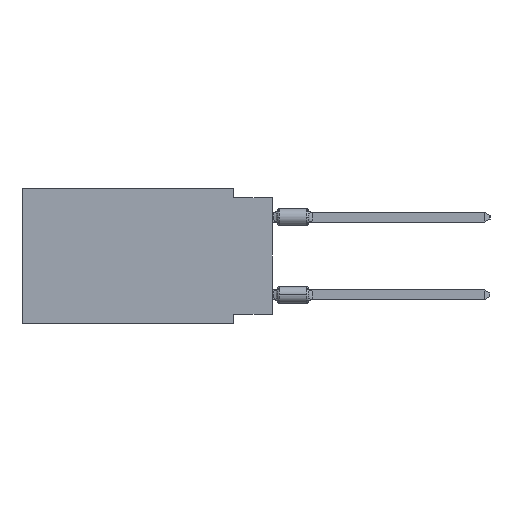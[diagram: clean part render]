
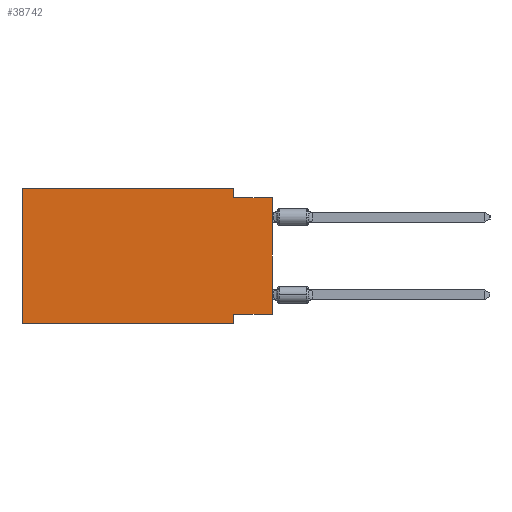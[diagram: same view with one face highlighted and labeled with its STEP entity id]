
A CAD part, left-side view. The second image highlights one B-rep face of the part: STEP entity #38742.
In plain terms, the highlighted planar face has unit normal (-1, 0, 0).
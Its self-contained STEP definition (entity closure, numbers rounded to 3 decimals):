
#643 = CARTESIAN_POINT ( 'NONE',  ( 0., 0., 0. ) ) ;
#2173 = EDGE_CURVE ( 'NONE', #18652, #46479, #44451, .T. ) ;
#4329 = LINE ( 'NONE', #19584, #11896 ) ;
#5005 = ORIENTED_EDGE ( 'NONE', *, *, #43931, .F. ) ;
#9536 = LINE ( 'NONE', #54314, #28170 ) ;
#9594 = ORIENTED_EDGE ( 'NONE', *, *, #46061, .F. ) ;
#10472 = VERTEX_POINT ( 'NONE', #29344 ) ;
#10672 = CARTESIAN_POINT ( 'NONE',  ( 0., 0., -8.255 ) ) ;
#11679 = DIRECTION ( 'NONE',  ( 0., -1., 0. ) ) ;
#11896 = VECTOR ( 'NONE', #43594, 1000. ) ;
#12153 = LINE ( 'NONE', #12464, #51001 ) ;
#12307 = CARTESIAN_POINT ( 'NONE',  ( 0., 2.54, 0. ) ) ;
#12359 = CARTESIAN_POINT ( 'NONE',  ( 0., 16.383, -8.89 ) ) ;
#12411 = VECTOR ( 'NONE', #62030, 1000. ) ;
#12464 = CARTESIAN_POINT ( 'NONE',  ( 0., 2.54, -8.89 ) ) ;
#12979 = VECTOR ( 'NONE', #44787, 1000. ) ;
#14026 = CARTESIAN_POINT ( 'NONE',  ( 0., 2.54, 0. ) ) ;
#14624 = CARTESIAN_POINT ( 'NONE',  ( 0., 16.383, 0. ) ) ;
#18652 = VERTEX_POINT ( 'NONE', #10672 ) ;
#19584 = CARTESIAN_POINT ( 'NONE',  ( 0., 0., -8.255 ) ) ;
#21296 = EDGE_CURVE ( 'NONE', #32334, #49037, #9536, .T. ) ;
#23120 = LINE ( 'NONE', #14026, #35484 ) ;
#23244 = CARTESIAN_POINT ( 'NONE',  ( 0., 2.54, -0.635 ) ) ;
#24096 = DIRECTION ( 'NONE',  ( 0., 0., -1. ) ) ;
#24366 = DIRECTION ( 'NONE',  ( 1., 0., 0. ) ) ;
#25274 = VERTEX_POINT ( 'NONE', #14624 ) ;
#25736 = ORIENTED_EDGE ( 'NONE', *, *, #50906, .F. ) ;
#26385 = EDGE_CURVE ( 'NONE', #18652, #10472, #4329, .T. ) ;
#26909 = LINE ( 'NONE', #47648, #53012 ) ;
#28170 = VECTOR ( 'NONE', #49128, 1000. ) ;
#28537 = CARTESIAN_POINT ( 'NONE',  ( 0., 0., -0.635 ) ) ;
#29253 = CARTESIAN_POINT ( 'NONE',  ( 0., 16.383, 0. ) ) ;
#29344 = CARTESIAN_POINT ( 'NONE',  ( 0., 2.54, -8.255 ) ) ;
#32278 = DIRECTION ( 'NONE',  ( 0., 0., -1. ) ) ;
#32334 = VERTEX_POINT ( 'NONE', #12359 ) ;
#32481 = CARTESIAN_POINT ( 'NONE',  ( 0., 16.383, 0. ) ) ;
#33287 = ORIENTED_EDGE ( 'NONE', *, *, #60538, .F. ) ;
#35484 = VECTOR ( 'NONE', #24096, 1000. ) ;
#38742 = ADVANCED_FACE ( 'NONE', ( #53575 ), #49689, .F. ) ;
#38971 = ORIENTED_EDGE ( 'NONE', *, *, #2173, .T. ) ;
#39308 = DIRECTION ( 'NONE',  ( 0., 0., 1. ) ) ;
#40540 = CARTESIAN_POINT ( 'NONE',  ( 0., 2.54, -8.89 ) ) ;
#40951 = EDGE_LOOP ( 'NONE', ( #38971, #5005, #33287, #25736, #63636, #56451, #9594, #52704 ) ) ;
#43594 = DIRECTION ( 'NONE',  ( 0., 1., 0. ) ) ;
#43931 = EDGE_CURVE ( 'NONE', #48147, #46479, #26909, .T. ) ;
#44451 = LINE ( 'NONE', #643, #12979 ) ;
#44787 = DIRECTION ( 'NONE',  ( 0., 0., 1. ) ) ;
#44822 = LINE ( 'NONE', #29253, #61423 ) ;
#44902 = EDGE_CURVE ( 'NONE', #32334, #25274, #44822, .T. ) ;
#45234 = VERTEX_POINT ( 'NONE', #12307 ) ;
#46061 = EDGE_CURVE ( 'NONE', #10472, #49037, #12153, .T. ) ;
#46479 = VERTEX_POINT ( 'NONE', #28537 ) ;
#47648 = CARTESIAN_POINT ( 'NONE',  ( 0., 0., -0.635 ) ) ;
#48147 = VERTEX_POINT ( 'NONE', #23244 ) ;
#49037 = VERTEX_POINT ( 'NONE', #40540 ) ;
#49040 = DIRECTION ( 'NONE',  ( 0., 0., -1. ) ) ;
#49128 = DIRECTION ( 'NONE',  ( 0., -1., 0. ) ) ;
#49689 = PLANE ( 'NONE',  #52358 ) ;
#50906 = EDGE_CURVE ( 'NONE', #25274, #45234, #62978, .T. ) ;
#51001 = VECTOR ( 'NONE', #32278, 1000. ) ;
#52358 = AXIS2_PLACEMENT_3D ( 'NONE', #53901, #24366, #49040 ) ;
#52704 = ORIENTED_EDGE ( 'NONE', *, *, #26385, .F. ) ;
#53012 = VECTOR ( 'NONE', #11679, 1000. ) ;
#53575 = FACE_OUTER_BOUND ( 'NONE', #40951, .T. ) ;
#53901 = CARTESIAN_POINT ( 'NONE',  ( 0., 16.383, 0. ) ) ;
#54314 = CARTESIAN_POINT ( 'NONE',  ( 0., 16.383, -8.89 ) ) ;
#56451 = ORIENTED_EDGE ( 'NONE', *, *, #21296, .T. ) ;
#60538 = EDGE_CURVE ( 'NONE', #45234, #48147, #23120, .T. ) ;
#61423 = VECTOR ( 'NONE', #39308, 1000. ) ;
#62030 = DIRECTION ( 'NONE',  ( 0., -1., 0. ) ) ;
#62978 = LINE ( 'NONE', #32481, #12411 ) ;
#63636 = ORIENTED_EDGE ( 'NONE', *, *, #44902, .F. ) ;
